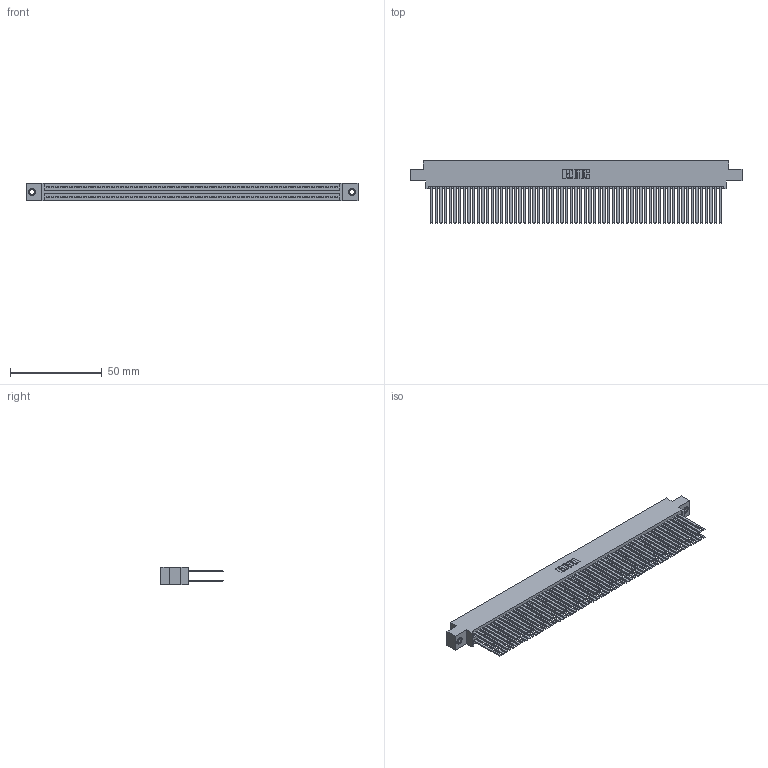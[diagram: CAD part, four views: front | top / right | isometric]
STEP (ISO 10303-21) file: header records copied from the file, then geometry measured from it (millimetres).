
FILE_DESCRIPTION (( 'STEP AP203' ), '1' );
FILE_NAME ('395-126-544-807.STEP', '2019-10-28T15:54:26', ( '' ), ( '' ), 'SwSTEP 2.0', 'SolidWorks 2016', '' );
FILE_SCHEMA (( 'CONFIG_CONTROL_DESIGN' ));
Length unit declared in the file: inch
Products named in the file (4): 345 Part_0.170 Offset - 0.156 Dia-TI; 345-292-001_345-293-144; 345-250-001_345-250-005-103; 395-126-544-807
Assembly tree (129 placements, depth 2):
  395-126-544-807
    345 Part_0.170 Offset - 0.156 Dia-TI
    345-292-001_345-293-144  x126
    345-250-001_345-250-005-103  x2
Bounding box: 181.23 x 33.96 x 9.4 mm (x, y, z)
Volume: 19439.1 mm3; surface area: 34489.1 mm2
Topology: 129 solids, 129 shells, 5734 faces, 16995 edges, 11154 vertices
Faces by surface type: plane 3770, cylinder 1948, cone 12, torus 4
Entity records: 47738 total; most frequent: CARTESIAN_POINT 7963, ORIENTED_EDGE 7890, DIRECTION 7019, EDGE_CURVE 3945, LINE 3545, VECTOR 3545, VERTEX_POINT 2624, AXIS2_PLACEMENT_3D 1737
